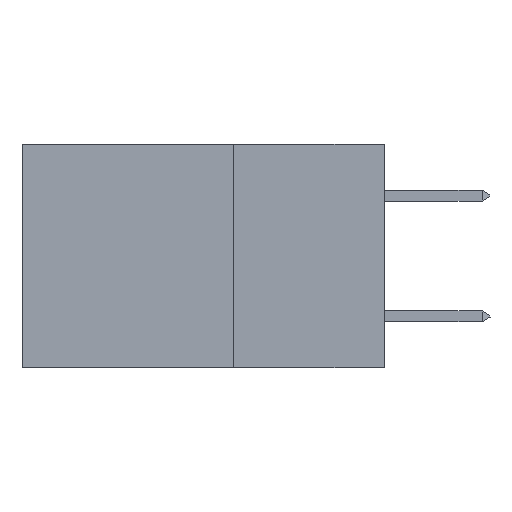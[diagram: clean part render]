
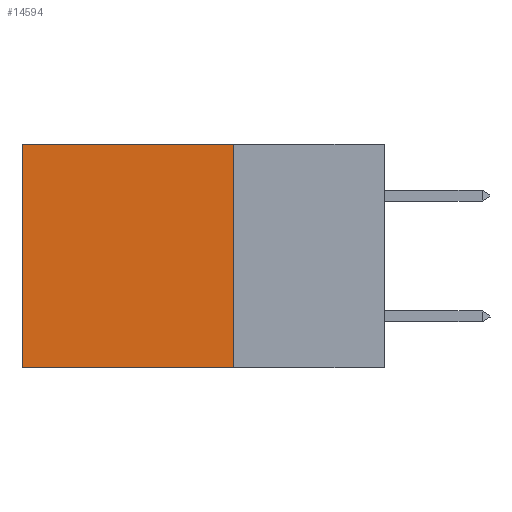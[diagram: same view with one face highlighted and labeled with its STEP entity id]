
A CAD part, left-side view. The second image highlights one B-rep face of the part: STEP entity #14594.
In plain terms, the highlighted planar face has unit normal (-1, 0, 0).
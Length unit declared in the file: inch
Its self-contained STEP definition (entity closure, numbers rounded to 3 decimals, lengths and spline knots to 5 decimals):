
#492 = ORIENTED_EDGE ( 'NONE', *, *, #1817, .F. ) ;
#1817 = EDGE_CURVE ( 'NONE', #6249, #17274, #8507, .T. ) ;
#3479 = PLANE ( 'NONE',  #20602 ) ;
#4465 = CARTESIAN_POINT ( 'NONE',  ( 0.2875, 0.25, -0.37 ) ) ;
#4639 = ORIENTED_EDGE ( 'NONE', *, *, #6629, .F. ) ;
#4852 = CARTESIAN_POINT ( 'NONE',  ( 0.2875, 0.25, 0. ) ) ;
#5454 = VERTEX_POINT ( 'NONE', #6897 ) ;
#6249 = VERTEX_POINT ( 'NONE', #15736 ) ;
#6287 = VERTEX_POINT ( 'NONE', #4852 ) ;
#6629 = EDGE_CURVE ( 'NONE', #6287, #6249, #9453, .T. ) ;
#6828 = EDGE_CURVE ( 'NONE', #6287, #5454, #9718, .T. ) ;
#6897 = CARTESIAN_POINT ( 'NONE',  ( 0.2875, 0.6, 0. ) ) ;
#8507 = LINE ( 'NONE', #4465, #22093 ) ;
#8619 = DIRECTION ( 'NONE',  ( 0., 1., 0. ) ) ;
#9453 = LINE ( 'NONE', #11269, #17917 ) ;
#9718 = LINE ( 'NONE', #22378, #19754 ) ;
#10765 = DIRECTION ( 'NONE',  ( 1., 0., 0. ) ) ;
#11090 = CARTESIAN_POINT ( 'NONE',  ( 0.2875, 0.6, 0. ) ) ;
#11269 = CARTESIAN_POINT ( 'NONE',  ( 0.2875, 0.25, 0. ) ) ;
#13226 = ORIENTED_EDGE ( 'NONE', *, *, #16076, .T. ) ;
#13675 = VECTOR ( 'NONE', #18368, 39.37008 ) ;
#14219 = EDGE_LOOP ( 'NONE', ( #13226, #492, #4639, #17316 ) ) ;
#14386 = CARTESIAN_POINT ( 'NONE',  ( 0.2875, 0.25, 0. ) ) ;
#14594 = ADVANCED_FACE ( 'NONE', ( #21970 ), #3479, .F. ) ;
#14874 = CARTESIAN_POINT ( 'NONE',  ( 0.2875, 0.6, -0.37 ) ) ;
#15736 = CARTESIAN_POINT ( 'NONE',  ( 0.2875, 0.25, -0.37 ) ) ;
#16076 = EDGE_CURVE ( 'NONE', #5454, #17274, #18437, .T. ) ;
#16730 = DIRECTION ( 'NONE',  ( 0., 0., -1. ) ) ;
#17274 = VERTEX_POINT ( 'NONE', #14874 ) ;
#17316 = ORIENTED_EDGE ( 'NONE', *, *, #6828, .T. ) ;
#17917 = VECTOR ( 'NONE', #16730, 39.37008 ) ;
#18368 = DIRECTION ( 'NONE',  ( 0., 0., -1. ) ) ;
#18437 = LINE ( 'NONE', #11090, #13675 ) ;
#18963 = DIRECTION ( 'NONE',  ( 0., 1., 0. ) ) ;
#19754 = VECTOR ( 'NONE', #18963, 39.37008 ) ;
#20602 = AXIS2_PLACEMENT_3D ( 'NONE', #14386, #10765, #23132 ) ;
#21970 = FACE_OUTER_BOUND ( 'NONE', #14219, .T. ) ;
#22093 = VECTOR ( 'NONE', #8619, 39.37008 ) ;
#22378 = CARTESIAN_POINT ( 'NONE',  ( 0.2875, 0.25, 0. ) ) ;
#23132 = DIRECTION ( 'NONE',  ( 0., 0., -1. ) ) ;
